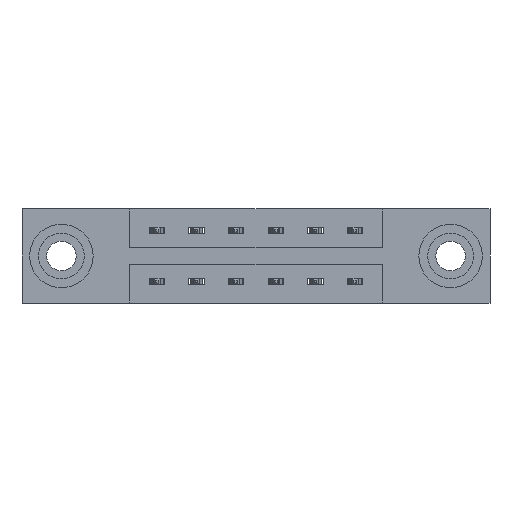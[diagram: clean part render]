
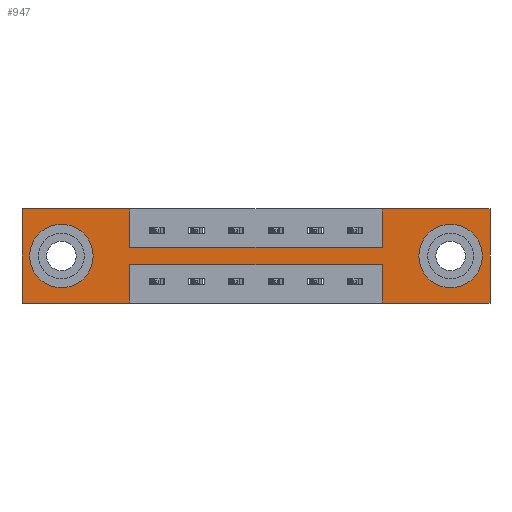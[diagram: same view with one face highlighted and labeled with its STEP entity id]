
A CAD part, front view. The second image highlights one B-rep face of the part: STEP entity #947.
In plain terms, the highlighted planar face has unit normal (0, -1, 0).
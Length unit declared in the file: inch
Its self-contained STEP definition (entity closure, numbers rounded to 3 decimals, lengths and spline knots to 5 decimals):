
#35 = ORIENTED_EDGE ( 'NONE', *, *, #5457, .T. ) ;
#45 = ORIENTED_EDGE ( 'NONE', *, *, #5195, .F. ) ;
#107 = VERTEX_POINT ( 'NONE', #3110 ) ;
#399 = EDGE_CURVE ( 'NONE', #2745, #6951, #4424, .T. ) ;
#460 = EDGE_CURVE ( 'NONE', #1310, #2757, #3941, .T. ) ;
#535 = CARTESIAN_POINT ( 'NONE',  ( 0.155, 0., -0.185 ) ) ;
#553 = LINE ( 'NONE', #3745, #2658 ) ;
#802 = CARTESIAN_POINT ( 'NONE',  ( 1.842, 0., -0.37 ) ) ;
#826 = EDGE_CURVE ( 'NONE', #2106, #6911, #1112, .T. ) ;
#894 = VECTOR ( 'NONE', #9017, 39.37008 ) ;
#947 = ADVANCED_FACE ( 'NONE', ( #8364, #3828, #9654 ), #2359, .T. ) ;
#990 = EDGE_CURVE ( 'NONE', #7113, #5844, #5383, .T. ) ;
#1001 = VECTOR ( 'NONE', #7109, 39.37008 ) ;
#1054 = DIRECTION ( 'NONE',  ( 0., 0., -1. ) ) ;
#1112 = LINE ( 'NONE', #3978, #2960 ) ;
#1115 = DIRECTION ( 'NONE',  ( 0., 0., -1. ) ) ;
#1159 = LINE ( 'NONE', #2135, #894 ) ;
#1310 = VERTEX_POINT ( 'NONE', #9228 ) ;
#1319 = DIRECTION ( 'NONE',  ( 0., 0., 1. ) ) ;
#1506 = DIRECTION ( 'NONE',  ( -1., 0., 0. ) ) ;
#1530 = CARTESIAN_POINT ( 'NONE',  ( 1.417, 0., -0.15 ) ) ;
#1626 = VERTEX_POINT ( 'NONE', #6987 ) ;
#1639 = DIRECTION ( 'NONE',  ( 0., -1., 0. ) ) ;
#1651 = CARTESIAN_POINT ( 'NONE',  ( 0.425, 0., 0. ) ) ;
#1869 = VECTOR ( 'NONE', #9517, 39.37008 ) ;
#1876 = CARTESIAN_POINT ( 'NONE',  ( 0.155, 0., -0.263 ) ) ;
#2106 = VERTEX_POINT ( 'NONE', #8718 ) ;
#2135 = CARTESIAN_POINT ( 'NONE',  ( 0., 0., -0.37 ) ) ;
#2166 = ORIENTED_EDGE ( 'NONE', *, *, #5272, .T. ) ;
#2323 = VECTOR ( 'NONE', #1506, 39.37008 ) ;
#2333 = DIRECTION ( 'NONE',  ( -1., 0., 0. ) ) ;
#2359 = PLANE ( 'NONE',  #8836 ) ;
#2416 = ORIENTED_EDGE ( 'NONE', *, *, #990, .F. ) ;
#2590 = EDGE_CURVE ( 'NONE', #3085, #5560, #7625, .T. ) ;
#2629 = AXIS2_PLACEMENT_3D ( 'NONE', #535, #5995, #1319 ) ;
#2658 = VECTOR ( 'NONE', #9055, 39.37008 ) ;
#2745 = VERTEX_POINT ( 'NONE', #7230 ) ;
#2757 = VERTEX_POINT ( 'NONE', #3499 ) ;
#2838 = CARTESIAN_POINT ( 'NONE',  ( 0.425, 0., -0.37 ) ) ;
#2924 = DIRECTION ( 'NONE',  ( 0., 0., 1. ) ) ;
#2960 = VECTOR ( 'NONE', #6517, 39.37008 ) ;
#2981 = DIRECTION ( 'NONE',  ( 1., 0., 0. ) ) ;
#3085 = VERTEX_POINT ( 'NONE', #2838 ) ;
#3086 = CARTESIAN_POINT ( 'NONE',  ( 0.425, 0., -0.22 ) ) ;
#3104 = LINE ( 'NONE', #5580, #1001 ) ;
#3110 = CARTESIAN_POINT ( 'NONE',  ( 1.417, 0., 0. ) ) ;
#3300 = EDGE_CURVE ( 'NONE', #5560, #5027, #553, .T. ) ;
#3305 = CIRCLE ( 'NONE', #9682, 0.078 ) ;
#3431 = CARTESIAN_POINT ( 'NONE',  ( 0., 0., 0. ) ) ;
#3499 = CARTESIAN_POINT ( 'NONE',  ( 1.687, 0., -0.107 ) ) ;
#3542 = LINE ( 'NONE', #7094, #5339 ) ;
#3621 = CARTESIAN_POINT ( 'NONE',  ( 0.155, 0., -0.185 ) ) ;
#3745 = CARTESIAN_POINT ( 'NONE',  ( 0., 0., 0. ) ) ;
#3828 = FACE_BOUND ( 'NONE', #6761, .T. ) ;
#3837 = VERTEX_POINT ( 'NONE', #1651 ) ;
#3941 = CIRCLE ( 'NONE', #6156, 0.078 ) ;
#3978 = CARTESIAN_POINT ( 'NONE',  ( 1.842, 0., 0. ) ) ;
#4041 = LINE ( 'NONE', #6011, #5847 ) ;
#4145 = VERTEX_POINT ( 'NONE', #1876 ) ;
#4180 = CARTESIAN_POINT ( 'NONE',  ( 0., 0., 0. ) ) ;
#4213 = LINE ( 'NONE', #3431, #1869 ) ;
#4231 = VERTEX_POINT ( 'NONE', #9040 ) ;
#4391 = CIRCLE ( 'NONE', #2629, 0.078 ) ;
#4392 = DIRECTION ( 'NONE',  ( 0., 0., 1. ) ) ;
#4424 = LINE ( 'NONE', #3086, #2323 ) ;
#4510 = ORIENTED_EDGE ( 'NONE', *, *, #7937, .F. ) ;
#4602 = DIRECTION ( 'NONE',  ( 0., 1., 0. ) ) ;
#4692 = EDGE_CURVE ( 'NONE', #5844, #107, #4041, .T. ) ;
#4760 = EDGE_LOOP ( 'NONE', ( #8553, #9018, #6897, #7134, #7849, #45, #6303, #2416, #4510, #4761, #6795, #7261 ) ) ;
#4761 = ORIENTED_EDGE ( 'NONE', *, *, #8546, .F. ) ;
#4762 = EDGE_CURVE ( 'NONE', #2757, #1310, #3305, .T. ) ;
#4885 = VECTOR ( 'NONE', #2981, 39.37008 ) ;
#5027 = VERTEX_POINT ( 'NONE', #4180 ) ;
#5044 = CARTESIAN_POINT ( 'NONE',  ( 0., 0., -0.37 ) ) ;
#5195 = EDGE_CURVE ( 'NONE', #107, #2106, #6899, .T. ) ;
#5272 = EDGE_CURVE ( 'NONE', #4145, #1626, #4391, .T. ) ;
#5323 = CARTESIAN_POINT ( 'NONE',  ( 0., 0., 0. ) ) ;
#5339 = VECTOR ( 'NONE', #1054, 39.37008 ) ;
#5383 = LINE ( 'NONE', #7773, #9411 ) ;
#5457 = EDGE_CURVE ( 'NONE', #1626, #4145, #7012, .T. ) ;
#5532 = DIRECTION ( 'NONE',  ( 0., 0., -1. ) ) ;
#5539 = CARTESIAN_POINT ( 'NONE',  ( 0.425, 0., -0.22 ) ) ;
#5560 = VERTEX_POINT ( 'NONE', #5044 ) ;
#5580 = CARTESIAN_POINT ( 'NONE',  ( 1.417, 0., -0.37 ) ) ;
#5581 = DIRECTION ( 'NONE',  ( 0., 1., 0. ) ) ;
#5650 = EDGE_CURVE ( 'NONE', #6951, #3085, #3542, .T. ) ;
#5844 = VERTEX_POINT ( 'NONE', #1530 ) ;
#5847 = VECTOR ( 'NONE', #2924, 39.37008 ) ;
#5995 = DIRECTION ( 'NONE',  ( 0., 1., 0. ) ) ;
#6011 = CARTESIAN_POINT ( 'NONE',  ( 1.417, 0., 0. ) ) ;
#6025 = CARTESIAN_POINT ( 'NONE',  ( 0., 0., -0.37 ) ) ;
#6156 = AXIS2_PLACEMENT_3D ( 'NONE', #7642, #5581, #5532 ) ;
#6264 = AXIS2_PLACEMENT_3D ( 'NONE', #3621, #8943, #4392 ) ;
#6303 = ORIENTED_EDGE ( 'NONE', *, *, #4692, .F. ) ;
#6517 = DIRECTION ( 'NONE',  ( 0., 0., -1. ) ) ;
#6641 = EDGE_CURVE ( 'NONE', #6911, #4231, #1159, .T. ) ;
#6740 = VECTOR ( 'NONE', #1115, 39.37008 ) ;
#6761 = EDGE_LOOP ( 'NONE', ( #35, #2166 ) ) ;
#6795 = ORIENTED_EDGE ( 'NONE', *, *, #3300, .F. ) ;
#6897 = ORIENTED_EDGE ( 'NONE', *, *, #8382, .F. ) ;
#6899 = LINE ( 'NONE', #5323, #4885 ) ;
#6911 = VERTEX_POINT ( 'NONE', #802 ) ;
#6951 = VERTEX_POINT ( 'NONE', #5539 ) ;
#6987 = CARTESIAN_POINT ( 'NONE',  ( 0.155, 0., -0.107 ) ) ;
#7012 = CIRCLE ( 'NONE', #6264, 0.078 ) ;
#7094 = CARTESIAN_POINT ( 'NONE',  ( 0.425, 0., -0.37 ) ) ;
#7109 = DIRECTION ( 'NONE',  ( 0., 0., 1. ) ) ;
#7113 = VERTEX_POINT ( 'NONE', #9470 ) ;
#7134 = ORIENTED_EDGE ( 'NONE', *, *, #6641, .F. ) ;
#7230 = CARTESIAN_POINT ( 'NONE',  ( 1.417, 0., -0.22 ) ) ;
#7261 = ORIENTED_EDGE ( 'NONE', *, *, #2590, .F. ) ;
#7329 = CARTESIAN_POINT ( 'NONE',  ( 0., 0., -0.37 ) ) ;
#7625 = LINE ( 'NONE', #7329, #9371 ) ;
#7642 = CARTESIAN_POINT ( 'NONE',  ( 1.687, 0., -0.185 ) ) ;
#7773 = CARTESIAN_POINT ( 'NONE',  ( 0.425, 0., -0.15 ) ) ;
#7841 = ORIENTED_EDGE ( 'NONE', *, *, #4762, .T. ) ;
#7849 = ORIENTED_EDGE ( 'NONE', *, *, #826, .F. ) ;
#7937 = EDGE_CURVE ( 'NONE', #3837, #7113, #8746, .T. ) ;
#8050 = CARTESIAN_POINT ( 'NONE',  ( 0.425, 0., 0. ) ) ;
#8364 = FACE_BOUND ( 'NONE', #8563, .T. ) ;
#8382 = EDGE_CURVE ( 'NONE', #4231, #2745, #3104, .T. ) ;
#8459 = DIRECTION ( 'NONE',  ( 1., 0., 0. ) ) ;
#8546 = EDGE_CURVE ( 'NONE', #5027, #3837, #4213, .T. ) ;
#8553 = ORIENTED_EDGE ( 'NONE', *, *, #5650, .F. ) ;
#8563 = EDGE_LOOP ( 'NONE', ( #7841, #9828 ) ) ;
#8718 = CARTESIAN_POINT ( 'NONE',  ( 1.842, 0., 0. ) ) ;
#8746 = LINE ( 'NONE', #8050, #6740 ) ;
#8836 = AXIS2_PLACEMENT_3D ( 'NONE', #6025, #1639, #9466 ) ;
#8943 = DIRECTION ( 'NONE',  ( 0., 1., 0. ) ) ;
#9017 = DIRECTION ( 'NONE',  ( -1., 0., 0. ) ) ;
#9018 = ORIENTED_EDGE ( 'NONE', *, *, #399, .F. ) ;
#9040 = CARTESIAN_POINT ( 'NONE',  ( 1.417, 0., -0.37 ) ) ;
#9055 = DIRECTION ( 'NONE',  ( 0., 0., 1. ) ) ;
#9139 = CARTESIAN_POINT ( 'NONE',  ( 1.687, 0., -0.185 ) ) ;
#9228 = CARTESIAN_POINT ( 'NONE',  ( 1.687, 0., -0.263 ) ) ;
#9371 = VECTOR ( 'NONE', #2333, 39.37008 ) ;
#9411 = VECTOR ( 'NONE', #8459, 39.37008 ) ;
#9466 = DIRECTION ( 'NONE',  ( 0., 0., -1. ) ) ;
#9470 = CARTESIAN_POINT ( 'NONE',  ( 0.425, 0., -0.15 ) ) ;
#9517 = DIRECTION ( 'NONE',  ( 1., 0., 0. ) ) ;
#9654 = FACE_OUTER_BOUND ( 'NONE', #4760, .T. ) ;
#9682 = AXIS2_PLACEMENT_3D ( 'NONE', #9139, #4602, #9888 ) ;
#9828 = ORIENTED_EDGE ( 'NONE', *, *, #460, .T. ) ;
#9888 = DIRECTION ( 'NONE',  ( 0., 0., -1. ) ) ;
